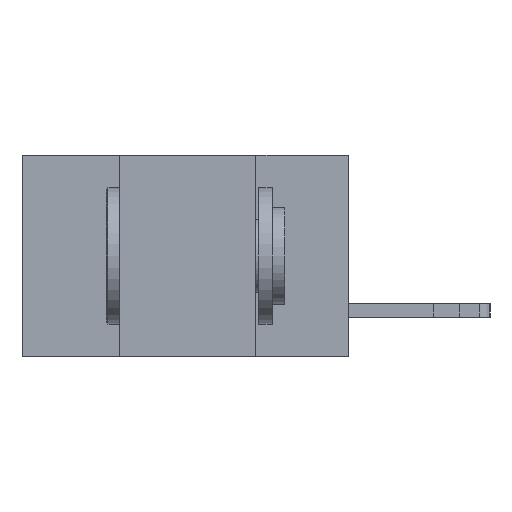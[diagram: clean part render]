
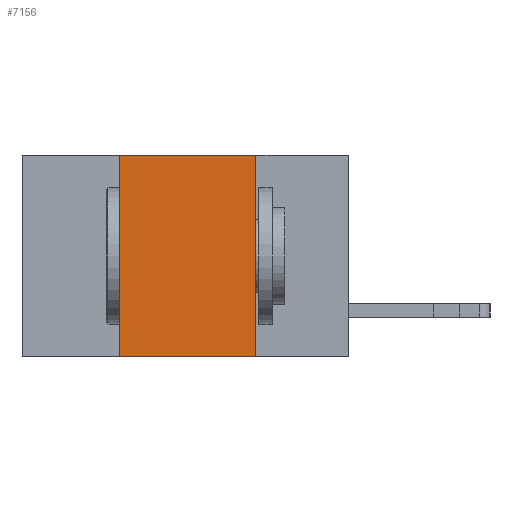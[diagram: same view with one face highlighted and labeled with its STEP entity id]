
A CAD part, left-side view. The second image highlights one B-rep face of the part: STEP entity #7156.
In plain terms, the highlighted planar face has unit normal (-1, 0, 0).
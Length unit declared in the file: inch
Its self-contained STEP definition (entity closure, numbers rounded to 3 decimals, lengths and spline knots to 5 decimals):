
#687 = LINE ( 'NONE', #14028, #17411 ) ;
#1127 = ORIENTED_EDGE ( 'NONE', *, *, #1539, .F. ) ;
#1377 = ORIENTED_EDGE ( 'NONE', *, *, #10917, .F. ) ;
#1539 = EDGE_CURVE ( 'NONE', #18410, #3874, #19145, .T. ) ;
#1618 = CARTESIAN_POINT ( 'NONE',  ( 0., 0.42, -0.37 ) ) ;
#1731 = VECTOR ( 'NONE', #18843, 39.37008 ) ;
#2391 = CARTESIAN_POINT ( 'NONE',  ( 0., 0.17, -0.37 ) ) ;
#2445 = ORIENTED_EDGE ( 'NONE', *, *, #9853, .F. ) ;
#2457 = ORIENTED_EDGE ( 'NONE', *, *, #11984, .T. ) ;
#3392 = CARTESIAN_POINT ( 'NONE',  ( 0., 0.42, 0. ) ) ;
#3874 = VERTEX_POINT ( 'NONE', #13691 ) ;
#4039 = DIRECTION ( 'NONE',  ( 0., -1., 0. ) ) ;
#4375 = DIRECTION ( 'NONE',  ( 0., 0., -1. ) ) ;
#5079 = DIRECTION ( 'NONE',  ( 0., 0., 1. ) ) ;
#5492 = VECTOR ( 'NONE', #5079, 39.37008 ) ;
#5633 = DIRECTION ( 'NONE',  ( 1., 0., 0. ) ) ;
#6281 = VERTEX_POINT ( 'NONE', #1618 ) ;
#7156 = ADVANCED_FACE ( 'NONE', ( #18372 ), #12021, .F. ) ;
#8281 = CARTESIAN_POINT ( 'NONE',  ( 0., 0.42, 0. ) ) ;
#9493 = LINE ( 'NONE', #17277, #1731 ) ;
#9853 = EDGE_CURVE ( 'NONE', #6281, #18410, #13965, .T. ) ;
#10774 = AXIS2_PLACEMENT_3D ( 'NONE', #15150, #5633, #16786 ) ;
#10917 = EDGE_CURVE ( 'NONE', #3874, #18640, #687, .T. ) ;
#11807 = EDGE_LOOP ( 'NONE', ( #1377, #1127, #2445, #2457 ) ) ;
#11984 = EDGE_CURVE ( 'NONE', #6281, #18640, #9493, .T. ) ;
#12021 = PLANE ( 'NONE',  #10774 ) ;
#13691 = CARTESIAN_POINT ( 'NONE',  ( 0., 0.17, 0. ) ) ;
#13965 = LINE ( 'NONE', #3392, #5492 ) ;
#14028 = CARTESIAN_POINT ( 'NONE',  ( 0., 0.17, 0. ) ) ;
#15150 = CARTESIAN_POINT ( 'NONE',  ( 0., 0.6, 0. ) ) ;
#16786 = DIRECTION ( 'NONE',  ( 0., 0., -1. ) ) ;
#17031 = CARTESIAN_POINT ( 'NONE',  ( 0., 0.6, 0. ) ) ;
#17277 = CARTESIAN_POINT ( 'NONE',  ( 0., 0.6, -0.37 ) ) ;
#17411 = VECTOR ( 'NONE', #4375, 39.37008 ) ;
#18372 = FACE_OUTER_BOUND ( 'NONE', #11807, .T. ) ;
#18410 = VERTEX_POINT ( 'NONE', #8281 ) ;
#18640 = VERTEX_POINT ( 'NONE', #2391 ) ;
#18666 = VECTOR ( 'NONE', #4039, 39.37008 ) ;
#18843 = DIRECTION ( 'NONE',  ( 0., -1., 0. ) ) ;
#19145 = LINE ( 'NONE', #17031, #18666 ) ;
